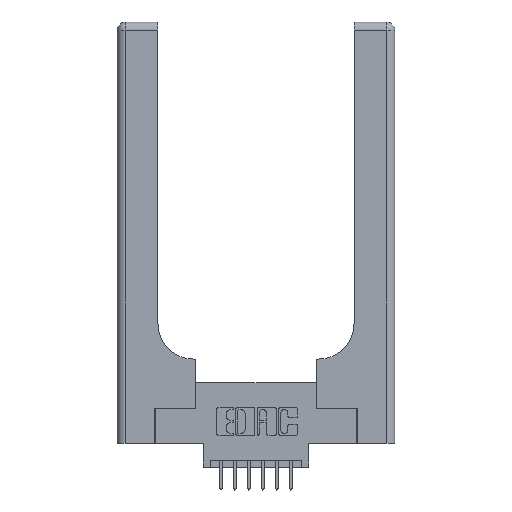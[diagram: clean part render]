
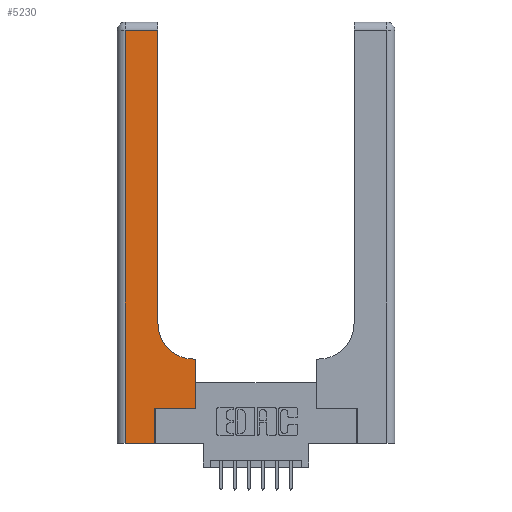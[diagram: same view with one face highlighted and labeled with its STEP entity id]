
A CAD part, top view. The second image highlights one B-rep face of the part: STEP entity #5230.
In plain terms, the highlighted planar face has unit normal (0, 0, 1).
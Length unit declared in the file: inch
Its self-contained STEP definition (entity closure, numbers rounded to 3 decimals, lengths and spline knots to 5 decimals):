
#359 = DIRECTION ( 'NONE',  ( -1., 0., 0. ) ) ;
#393 = LINE ( 'NONE', #5438, #4556 ) ;
#517 = ORIENTED_EDGE ( 'NONE', *, *, #5596, .T. ) ;
#669 = ORIENTED_EDGE ( 'NONE', *, *, #1418, .T. ) ;
#893 = EDGE_CURVE ( 'NONE', #14237, #2998, #4893, .T. ) ;
#1048 = LINE ( 'NONE', #8822, #7897 ) ;
#1098 = VERTEX_POINT ( 'NONE', #4752 ) ;
#1418 = EDGE_CURVE ( 'NONE', #14296, #14237, #9442, .T. ) ;
#1807 = EDGE_CURVE ( 'NONE', #11130, #5515, #393, .T. ) ;
#1837 = VECTOR ( 'NONE', #5593, 39.37008 ) ;
#1905 = VERTEX_POINT ( 'NONE', #12619 ) ;
#1980 = DIRECTION ( 'NONE',  ( 0., 0., -1. ) ) ;
#2049 = DIRECTION ( 'NONE',  ( -1., 0., 0. ) ) ;
#2170 = DIRECTION ( 'NONE',  ( 0., 1., 0. ) ) ;
#2364 = VECTOR ( 'NONE', #2049, 39.37008 ) ;
#2444 = ORIENTED_EDGE ( 'NONE', *, *, #1807, .T. ) ;
#2615 = CARTESIAN_POINT ( 'NONE',  ( 0.5585, 0.25, 0.37 ) ) ;
#2927 = CARTESIAN_POINT ( 'NONE',  ( 0.06, 2.94, 0.37 ) ) ;
#2998 = VERTEX_POINT ( 'NONE', #2927 ) ;
#3069 = DIRECTION ( 'NONE',  ( 0., 1., 0. ) ) ;
#3785 = ORIENTED_EDGE ( 'NONE', *, *, #893, .T. ) ;
#3938 = DIRECTION ( 'NONE',  ( 1., 0., 0. ) ) ;
#4071 = EDGE_CURVE ( 'NONE', #2998, #11130, #14761, .T. ) ;
#4142 = LINE ( 'NONE', #7986, #2364 ) ;
#4556 = VECTOR ( 'NONE', #10086, 39.37008 ) ;
#4752 = CARTESIAN_POINT ( 'NONE',  ( 0.5585, 0.6, 0.37 ) ) ;
#4758 = CARTESIAN_POINT ( 'NONE',  ( 0.269, 0., 0.37 ) ) ;
#4893 = LINE ( 'NONE', #13569, #1837 ) ;
#5229 = ORIENTED_EDGE ( 'NONE', *, *, #10160, .T. ) ;
#5230 = ADVANCED_FACE ( 'NONE', ( #12575 ), #14175, .F. ) ;
#5340 = AXIS2_PLACEMENT_3D ( 'NONE', #10765, #10857, #359 ) ;
#5438 = CARTESIAN_POINT ( 'NONE',  ( 0., 0., 0.37 ) ) ;
#5443 = LINE ( 'NONE', #14021, #10011 ) ;
#5515 = VERTEX_POINT ( 'NONE', #4758 ) ;
#5593 = DIRECTION ( 'NONE',  ( -1., 0., 0. ) ) ;
#5596 = EDGE_CURVE ( 'NONE', #10502, #1098, #9658, .T. ) ;
#5905 = DIRECTION ( 'NONE',  ( 0., 1., 0. ) ) ;
#6101 = CARTESIAN_POINT ( 'NONE',  ( 0.06, 0., 0.37 ) ) ;
#6340 = CIRCLE ( 'NONE', #11642, 0.25 ) ;
#6821 = ORIENTED_EDGE ( 'NONE', *, *, #4071, .T. ) ;
#6857 = EDGE_CURVE ( 'NONE', #10625, #10502, #5443, .T. ) ;
#7578 = CARTESIAN_POINT ( 'NONE',  ( 0.5415, 0.85, 0.37 ) ) ;
#7897 = VECTOR ( 'NONE', #3069, 39.37008 ) ;
#7986 = CARTESIAN_POINT ( 'NONE',  ( 0.2915, 0.6, 0.37 ) ) ;
#8346 = DIRECTION ( 'NONE',  ( 0., -1., 0. ) ) ;
#8822 = CARTESIAN_POINT ( 'NONE',  ( 0.269, 0., 0.37 ) ) ;
#9353 = ORIENTED_EDGE ( 'NONE', *, *, #11938, .T. ) ;
#9442 = LINE ( 'NONE', #13690, #11080 ) ;
#9658 = LINE ( 'NONE', #2615, #14705 ) ;
#9799 = EDGE_LOOP ( 'NONE', ( #669, #3785, #6821, #2444, #5229, #10559, #517, #13967, #9353 ) ) ;
#9876 = VECTOR ( 'NONE', #8346, 39.37008 ) ;
#10011 = VECTOR ( 'NONE', #3938, 39.37008 ) ;
#10086 = DIRECTION ( 'NONE',  ( 1., 0., 0. ) ) ;
#10160 = EDGE_CURVE ( 'NONE', #5515, #10625, #1048, .T. ) ;
#10284 = CARTESIAN_POINT ( 'NONE',  ( 0.2915, 2.94, 0.37 ) ) ;
#10502 = VERTEX_POINT ( 'NONE', #11745 ) ;
#10559 = ORIENTED_EDGE ( 'NONE', *, *, #6857, .T. ) ;
#10625 = VERTEX_POINT ( 'NONE', #12878 ) ;
#10765 = CARTESIAN_POINT ( 'NONE',  ( 0., 3., 0.37 ) ) ;
#10857 = DIRECTION ( 'NONE',  ( 0., 0., -1. ) ) ;
#10976 = CARTESIAN_POINT ( 'NONE',  ( 0.2915, 0.85, 0.37 ) ) ;
#11080 = VECTOR ( 'NONE', #2170, 39.37008 ) ;
#11130 = VERTEX_POINT ( 'NONE', #6101 ) ;
#11642 = AXIS2_PLACEMENT_3D ( 'NONE', #7578, #1980, #12349 ) ;
#11745 = CARTESIAN_POINT ( 'NONE',  ( 0.5585, 0.25, 0.37 ) ) ;
#11938 = EDGE_CURVE ( 'NONE', #1905, #14296, #6340, .T. ) ;
#12349 = DIRECTION ( 'NONE',  ( 1., 0., 0. ) ) ;
#12575 = FACE_OUTER_BOUND ( 'NONE', #9799, .T. ) ;
#12619 = CARTESIAN_POINT ( 'NONE',  ( 0.5415, 0.6, 0.37 ) ) ;
#12820 = CARTESIAN_POINT ( 'NONE',  ( 0.06, 3., 0.37 ) ) ;
#12878 = CARTESIAN_POINT ( 'NONE',  ( 0.269, 0.25, 0.37 ) ) ;
#13157 = EDGE_CURVE ( 'NONE', #1098, #1905, #4142, .T. ) ;
#13569 = CARTESIAN_POINT ( 'NONE',  ( 0., 2.94, 0.37 ) ) ;
#13690 = CARTESIAN_POINT ( 'NONE',  ( 0.2915, 3., 0.37 ) ) ;
#13967 = ORIENTED_EDGE ( 'NONE', *, *, #13157, .T. ) ;
#14021 = CARTESIAN_POINT ( 'NONE',  ( 0.269, 0.25, 0.37 ) ) ;
#14175 = PLANE ( 'NONE',  #5340 ) ;
#14237 = VERTEX_POINT ( 'NONE', #10284 ) ;
#14296 = VERTEX_POINT ( 'NONE', #10976 ) ;
#14705 = VECTOR ( 'NONE', #5905, 39.37008 ) ;
#14761 = LINE ( 'NONE', #12820, #9876 ) ;
